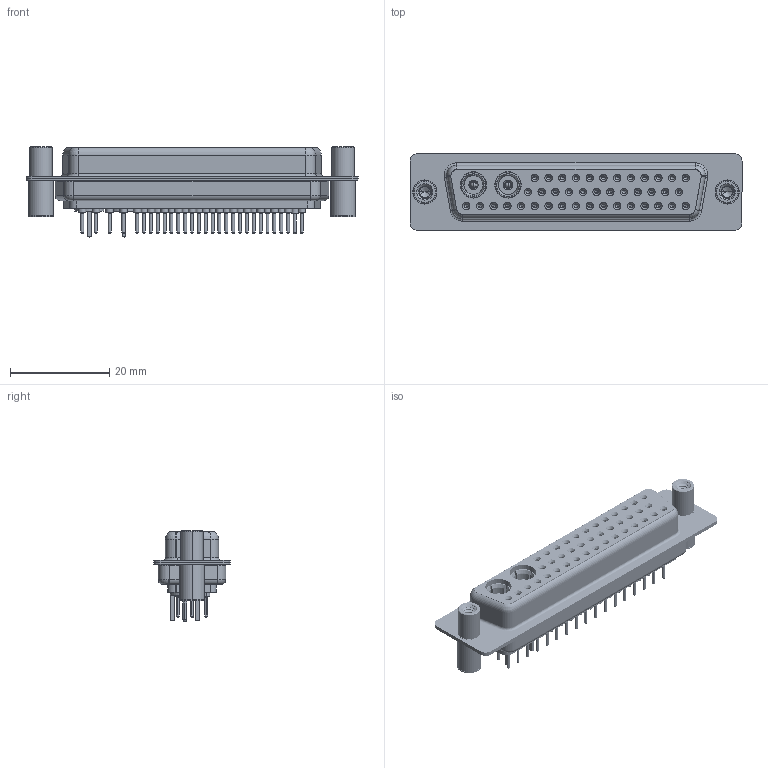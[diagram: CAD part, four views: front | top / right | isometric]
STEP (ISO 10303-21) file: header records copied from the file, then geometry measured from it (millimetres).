
FILE_DESCRIPTION (( 'STEP AP203' ), '1' );
FILE_NAME ('628-43W2624-5N4.STEP', '2019-06-26T21:18:27', ( '' ), ( '' ), 'SwSTEP 2.0', 'SolidWorks 2016', '' );
FILE_SCHEMA (( 'CONFIG_CONTROL_DESIGN' ));
Length unit declared in the file: millimetre
Products named in the file (13): Co-Ax Plug_Straight PC Tail; Pin_Str; 628Combo Threaded Standoff and Board Spacer_4; Locking Collar; Insulator Pin_Straight PC Tail; 628Combo Contact Row 1_24; Co-Ax Plug Assy_St; 628Combo Contact Row 3_24; 628Combo Housing_43W2; 628Combo Shell Front_50 Contacts; 628-43W2624-5N4; 628Combo Contact Row 2_24; 628Combo Shell Rear_50 Contacts
Assembly tree (52 placements, depth 3):
  628-43W2624-5N4
    628Combo Housing_43W2
    628Combo Shell Front_50 Contacts
    628Combo Shell Rear_50 Contacts
    628Combo Threaded Standoff and Board Spacer_4  x2
    628Combo Contact Row 1_24  x12
    628Combo Contact Row 2_24  x12
    628Combo Contact Row 3_24  x17
    Co-Ax Plug Assy_St  x2
      Co-Ax Plug_Straight PC Tail
      Insulator Pin_Straight PC Tail
      Pin_Str
      Locking Collar
Bounding box: 67 x 15.4 x 18.35 mm (x, y, z)
Volume: 7217.2 mm3; surface area: 15510.4 mm2
Topology: 54 solids, 54 shells, 2874 faces, 6687 edges, 4110 vertices
Faces by surface type: cylinder 1058, plane 802, torus 643, cone 347, bspline 16, sphere 8
Entity records: 35769 total; most frequent: CARTESIAN_POINT 7785, DIRECTION 5901, ORIENTED_EDGE 4920, AXIS2_PLACEMENT_3D 2487, EDGE_CURVE 2460, VERTEX_POINT 1561, CIRCLE 1359, EDGE_LOOP 1341
